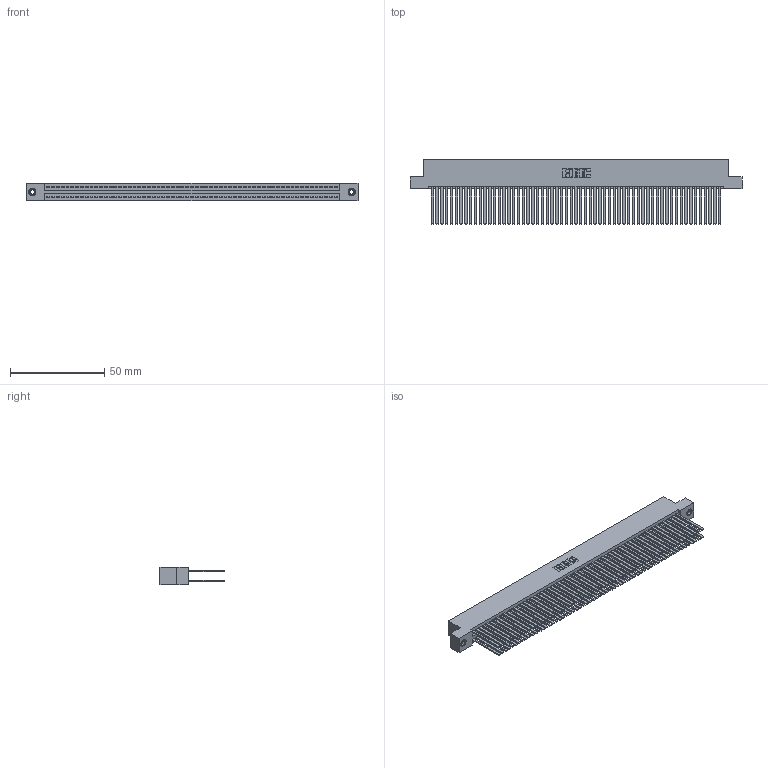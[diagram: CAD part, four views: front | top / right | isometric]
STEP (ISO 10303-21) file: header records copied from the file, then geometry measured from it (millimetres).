
FILE_DESCRIPTION (( 'STEP AP203' ), '1' );
FILE_NAME ('845-122-544-208.STEP', '2018-11-21T12:17:21', ( '' ), ( '' ), 'SwSTEP 2.0', 'SolidWorks 2016', '' );
FILE_SCHEMA (( 'CONFIG_CONTROL_DESIGN' ));
Length unit declared in the file: inch
Products named in the file (4): 845 Part_Flush Mounting Lugs - 0.156 Dia-TI; 345-292-001_345-293-144; 345-250-001_345-250-003-102; 845-122-544-208
Assembly tree (125 placements, depth 2):
  845-122-544-208
    845 Part_Flush Mounting Lugs - 0.156 Dia-TI
    345-292-001_345-293-144  x122
    345-250-001_345-250-003-102  x2
Bounding box: 176.15 x 33.96 x 9.4 mm (x, y, z)
Volume: 18991.4 mm3; surface area: 33466.3 mm2
Topology: 125 solids, 125 shells, 5554 faces, 16459 edges, 10802 vertices
Faces by surface type: plane 3650, cylinder 1888, cone 12, torus 4
Entity records: 46306 total; most frequent: CARTESIAN_POINT 7723, ORIENTED_EDGE 7650, DIRECTION 6811, EDGE_CURVE 3825, LINE 3433, VECTOR 3433, VERTEX_POINT 2544, AXIS2_PLACEMENT_3D 1689
